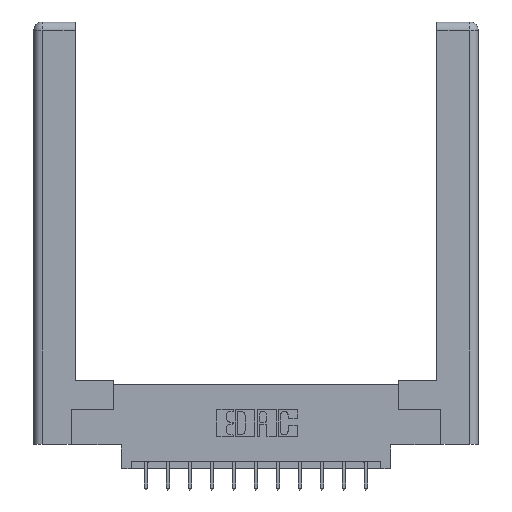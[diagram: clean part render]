
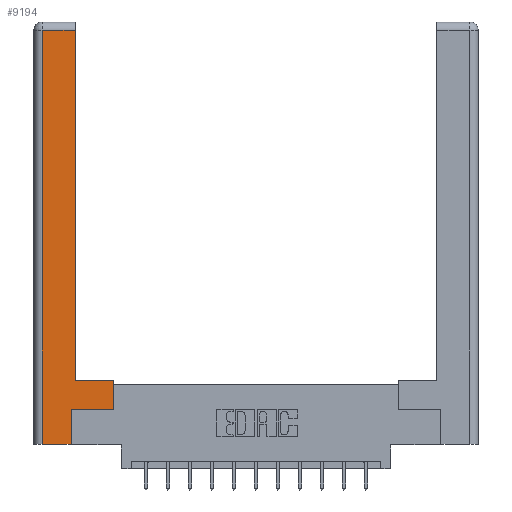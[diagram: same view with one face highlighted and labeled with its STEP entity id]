
A CAD part, top view. The second image highlights one B-rep face of the part: STEP entity #9194.
In plain terms, the highlighted planar face has unit normal (0, 0, 1).
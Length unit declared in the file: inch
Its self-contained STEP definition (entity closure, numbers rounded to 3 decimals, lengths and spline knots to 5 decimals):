
#81 = LINE ( 'NONE', #1517, #6002 ) ;
#357 = VECTOR ( 'NONE', #5790, 39.37008 ) ;
#464 = LINE ( 'NONE', #10002, #9918 ) ;
#465 = EDGE_CURVE ( 'NONE', #10309, #9922, #81, .T. ) ;
#1024 = VERTEX_POINT ( 'NONE', #1197 ) ;
#1197 = CARTESIAN_POINT ( 'NONE',  ( 0.295, 2.94, 0. ) ) ;
#1302 = CARTESIAN_POINT ( 'NONE',  ( 0.565, 0.245, 0. ) ) ;
#1476 = CARTESIAN_POINT ( 'NONE',  ( 0.265, 0.245, 0. ) ) ;
#1517 = CARTESIAN_POINT ( 'NONE',  ( 0.295, 0.45, 0. ) ) ;
#1792 = CARTESIAN_POINT ( 'NONE',  ( 0.0615, 2.94, 0. ) ) ;
#1937 = VERTEX_POINT ( 'NONE', #4057 ) ;
#2309 = AXIS2_PLACEMENT_3D ( 'NONE', #14999, #9198, #12598 ) ;
#2468 = FACE_OUTER_BOUND ( 'NONE', #5300, .T. ) ;
#2506 = EDGE_CURVE ( 'NONE', #1937, #13285, #8149, .T. ) ;
#3071 = VECTOR ( 'NONE', #8548, 39.37008 ) ;
#3078 = ORIENTED_EDGE ( 'NONE', *, *, #2506, .T. ) ;
#3362 = DIRECTION ( 'NONE',  ( 1., 0., 0. ) ) ;
#3369 = ORIENTED_EDGE ( 'NONE', *, *, #14256, .T. ) ;
#3442 = ORIENTED_EDGE ( 'NONE', *, *, #7583, .T. ) ;
#4057 = CARTESIAN_POINT ( 'NONE',  ( 0.265, 0., 0. ) ) ;
#4577 = VECTOR ( 'NONE', #4866, 39.37008 ) ;
#4824 = VERTEX_POINT ( 'NONE', #8296 ) ;
#4832 = CARTESIAN_POINT ( 'NONE',  ( 0.265, 0., 0. ) ) ;
#4866 = DIRECTION ( 'NONE',  ( -1., 0., 0. ) ) ;
#5151 = DIRECTION ( 'NONE',  ( 0., 1., 0. ) ) ;
#5300 = EDGE_LOOP ( 'NONE', ( #14310, #9251, #3442, #5797, #3078, #11885, #3369, #11586 ) ) ;
#5790 = DIRECTION ( 'NONE',  ( 0., -1., 0. ) ) ;
#5797 = ORIENTED_EDGE ( 'NONE', *, *, #7109, .T. ) ;
#5806 = EDGE_CURVE ( 'NONE', #1024, #14823, #6789, .T. ) ;
#5872 = LINE ( 'NONE', #11679, #357 ) ;
#5914 = VECTOR ( 'NONE', #14422, 39.37008 ) ;
#6002 = VECTOR ( 'NONE', #10786, 39.37008 ) ;
#6228 = CARTESIAN_POINT ( 'NONE',  ( 0.0615, 0., 0. ) ) ;
#6321 = VERTEX_POINT ( 'NONE', #6228 ) ;
#6789 = LINE ( 'NONE', #7012, #4577 ) ;
#7012 = CARTESIAN_POINT ( 'NONE',  ( 0.0615, 2.94, 0. ) ) ;
#7109 = EDGE_CURVE ( 'NONE', #6321, #1937, #12475, .T. ) ;
#7583 = EDGE_CURVE ( 'NONE', #14823, #6321, #5872, .T. ) ;
#7903 = EDGE_CURVE ( 'NONE', #9922, #1024, #12479, .T. ) ;
#8149 = LINE ( 'NONE', #1476, #5914 ) ;
#8296 = CARTESIAN_POINT ( 'NONE',  ( 0.565, 0.245, 0. ) ) ;
#8368 = CARTESIAN_POINT ( 'NONE',  ( 0.565, 0.45, 0. ) ) ;
#8548 = DIRECTION ( 'NONE',  ( 1., 0., 0. ) ) ;
#8848 = PLANE ( 'NONE',  #2309 ) ;
#9194 = ADVANCED_FACE ( 'NONE', ( #2468 ), #8848, .F. ) ;
#9198 = DIRECTION ( 'NONE',  ( 0., 0., -1. ) ) ;
#9251 = ORIENTED_EDGE ( 'NONE', *, *, #5806, .T. ) ;
#9918 = VECTOR ( 'NONE', #5151, 39.37008 ) ;
#9922 = VERTEX_POINT ( 'NONE', #13351 ) ;
#9956 = LINE ( 'NONE', #1302, #10693 ) ;
#10002 = CARTESIAN_POINT ( 'NONE',  ( 0.565, 0.45, 0. ) ) ;
#10309 = VERTEX_POINT ( 'NONE', #8368 ) ;
#10693 = VECTOR ( 'NONE', #3362, 39.37008 ) ;
#10786 = DIRECTION ( 'NONE',  ( -1., 0., 0. ) ) ;
#11423 = CARTESIAN_POINT ( 'NONE',  ( 0.265, 0.245, 0. ) ) ;
#11426 = CARTESIAN_POINT ( 'NONE',  ( 0.295, 3., 0. ) ) ;
#11586 = ORIENTED_EDGE ( 'NONE', *, *, #465, .T. ) ;
#11679 = CARTESIAN_POINT ( 'NONE',  ( 0.0615, 0., 0. ) ) ;
#11885 = ORIENTED_EDGE ( 'NONE', *, *, #14106, .T. ) ;
#12475 = LINE ( 'NONE', #4832, #3071 ) ;
#12479 = LINE ( 'NONE', #11426, #14166 ) ;
#12598 = DIRECTION ( 'NONE',  ( -1., 0., 0. ) ) ;
#13285 = VERTEX_POINT ( 'NONE', #11423 ) ;
#13351 = CARTESIAN_POINT ( 'NONE',  ( 0.295, 0.45, 0. ) ) ;
#13641 = DIRECTION ( 'NONE',  ( 0., 1., 0. ) ) ;
#14106 = EDGE_CURVE ( 'NONE', #13285, #4824, #9956, .T. ) ;
#14166 = VECTOR ( 'NONE', #13641, 39.37008 ) ;
#14256 = EDGE_CURVE ( 'NONE', #4824, #10309, #464, .T. ) ;
#14310 = ORIENTED_EDGE ( 'NONE', *, *, #7903, .T. ) ;
#14422 = DIRECTION ( 'NONE',  ( 0., 1., 0. ) ) ;
#14823 = VERTEX_POINT ( 'NONE', #1792 ) ;
#14999 = CARTESIAN_POINT ( 'NONE',  ( 0., 0., 0. ) ) ;
